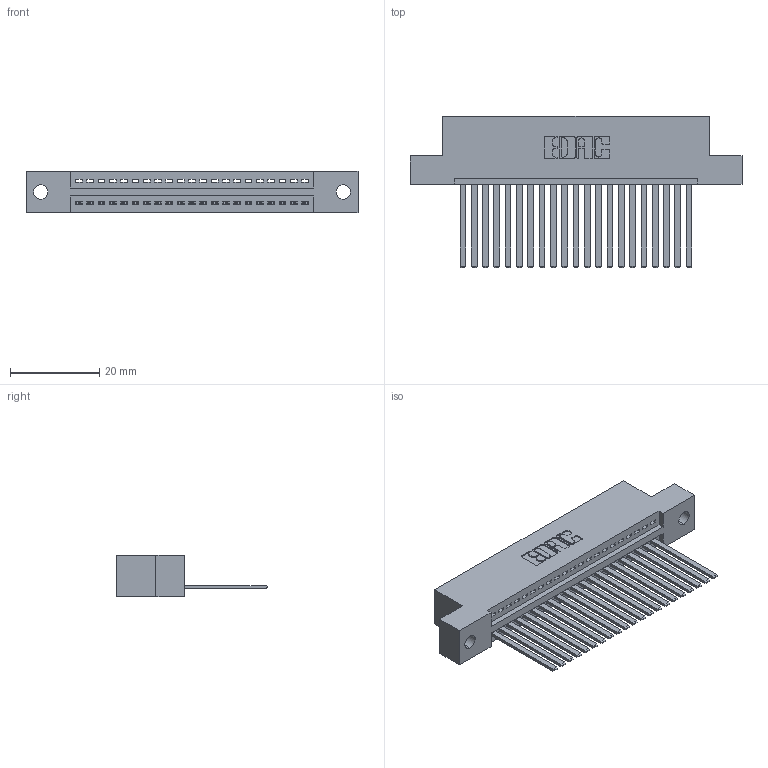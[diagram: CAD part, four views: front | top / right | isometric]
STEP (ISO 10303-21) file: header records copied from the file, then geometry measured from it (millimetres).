
FILE_DESCRIPTION (( 'STEP AP203' ), '1' );
FILE_NAME ('345-021-544-102.STEP', '2018-08-20T09:44:46', ( '' ), ( '' ), 'SwSTEP 2.0', 'SolidWorks 2016', '' );
FILE_SCHEMA (( 'CONFIG_CONTROL_DESIGN' ));
Length unit declared in the file: inch
Products named in the file (3): 345 Part_Flush Mounting Lugs - 0.128 Dia; 345-292-001_345-293-144; 345-021-544-102
Assembly tree (22 placements, depth 2):
  345-021-544-102
    345 Part_Flush Mounting Lugs - 0.128 Dia
    345-292-001_345-293-144  x21
Bounding box: 74.55 x 33.96 x 9.4 mm (x, y, z)
Volume: 7115.2 mm3; surface area: 9628.7 mm2
Topology: 22 solids, 22 shells, 1218 faces, 3659 edges, 2410 vertices
Faces by surface type: plane 836, cylinder 382
Entity records: 18451 total; most frequent: CARTESIAN_POINT 3203, ORIENTED_EDGE 3158, DIRECTION 2825, EDGE_CURVE 1579, LINE 1367, VECTOR 1367, VERTEX_POINT 1050, AXIS2_PLACEMENT_3D 729
